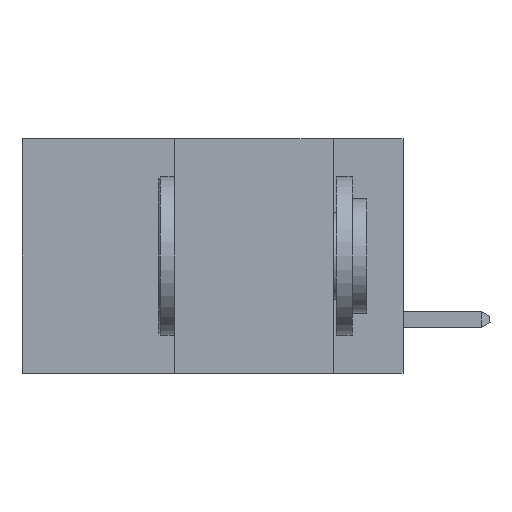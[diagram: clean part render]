
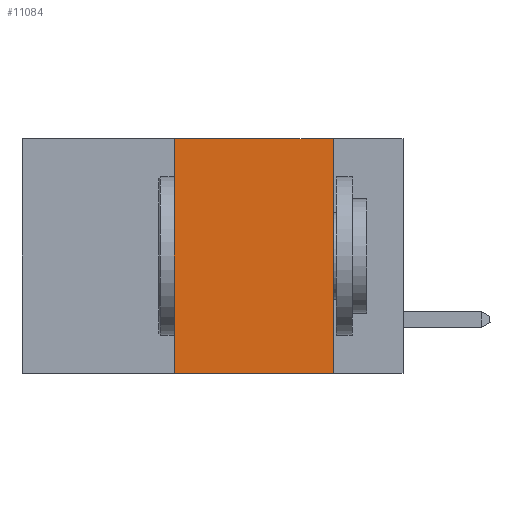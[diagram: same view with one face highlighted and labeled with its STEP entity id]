
A CAD part, left-side view. The second image highlights one B-rep face of the part: STEP entity #11084.
In plain terms, the highlighted planar face has unit normal (-1, 0, 0).
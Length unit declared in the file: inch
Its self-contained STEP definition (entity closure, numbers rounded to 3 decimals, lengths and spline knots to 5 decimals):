
#4 = ORIENTED_EDGE ( 'NONE', *, *, #16193, .F. ) ;
#45 = CARTESIAN_POINT ( 'NONE',  ( 0., 0.11, 0. ) ) ;
#200 = VECTOR ( 'NONE', #10488, 39.37008 ) ;
#1175 = CARTESIAN_POINT ( 'NONE',  ( 0., 0.11, 0. ) ) ;
#3515 = DIRECTION ( 'NONE',  ( 0., 0., 1. ) ) ;
#3621 = LINE ( 'NONE', #16487, #200 ) ;
#4766 = EDGE_CURVE ( 'NONE', #11542, #15398, #5314, .T. ) ;
#5314 = LINE ( 'NONE', #1175, #6288 ) ;
#6288 = VECTOR ( 'NONE', #18122, 39.37008 ) ;
#7239 = FACE_OUTER_BOUND ( 'NONE', #10882, .T. ) ;
#8084 = CARTESIAN_POINT ( 'NONE',  ( 0., 0.36, 0. ) ) ;
#8525 = VERTEX_POINT ( 'NONE', #18811 ) ;
#8605 = EDGE_CURVE ( 'NONE', #8525, #11080, #13870, .T. ) ;
#8638 = DIRECTION ( 'NONE',  ( 0., -1., 0. ) ) ;
#9585 = EDGE_CURVE ( 'NONE', #8525, #15398, #15960, .T. ) ;
#10189 = CARTESIAN_POINT ( 'NONE',  ( 0., 0.6, -0.37 ) ) ;
#10488 = DIRECTION ( 'NONE',  ( 0., -1., 0. ) ) ;
#10882 = EDGE_LOOP ( 'NONE', ( #12629, #4, #13618, #13754 ) ) ;
#11080 = VERTEX_POINT ( 'NONE', #17737 ) ;
#11084 = ADVANCED_FACE ( 'NONE', ( #7239 ), #17799, .F. ) ;
#11542 = VERTEX_POINT ( 'NONE', #45 ) ;
#11660 = CARTESIAN_POINT ( 'NONE',  ( 0., 0.6, 0. ) ) ;
#11864 = VECTOR ( 'NONE', #8638, 39.37008 ) ;
#12629 = ORIENTED_EDGE ( 'NONE', *, *, #4766, .F. ) ;
#13003 = DIRECTION ( 'NONE',  ( 0., 0., -1. ) ) ;
#13618 = ORIENTED_EDGE ( 'NONE', *, *, #8605, .F. ) ;
#13754 = ORIENTED_EDGE ( 'NONE', *, *, #9585, .T. ) ;
#13870 = LINE ( 'NONE', #8084, #18490 ) ;
#15398 = VERTEX_POINT ( 'NONE', #17602 ) ;
#15960 = LINE ( 'NONE', #10189, #11864 ) ;
#16193 = EDGE_CURVE ( 'NONE', #11080, #11542, #3621, .T. ) ;
#16296 = DIRECTION ( 'NONE',  ( 1., 0., 0. ) ) ;
#16487 = CARTESIAN_POINT ( 'NONE',  ( 0., 0.6, 0. ) ) ;
#17314 = AXIS2_PLACEMENT_3D ( 'NONE', #11660, #16296, #13003 ) ;
#17602 = CARTESIAN_POINT ( 'NONE',  ( 0., 0.11, -0.37 ) ) ;
#17737 = CARTESIAN_POINT ( 'NONE',  ( 0., 0.36, 0. ) ) ;
#17799 = PLANE ( 'NONE',  #17314 ) ;
#18122 = DIRECTION ( 'NONE',  ( 0., 0., -1. ) ) ;
#18490 = VECTOR ( 'NONE', #3515, 39.37008 ) ;
#18811 = CARTESIAN_POINT ( 'NONE',  ( 0., 0.36, -0.37 ) ) ;
